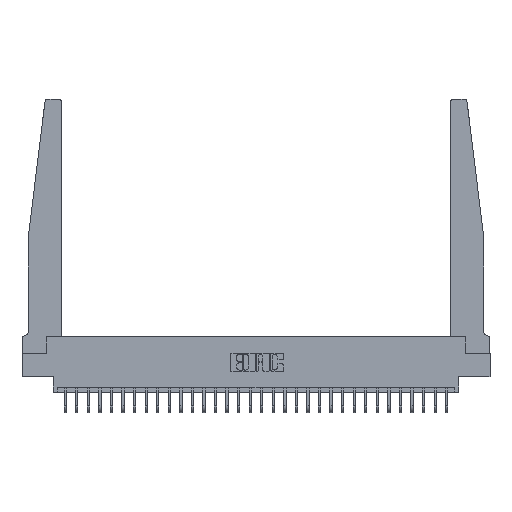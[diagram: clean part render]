
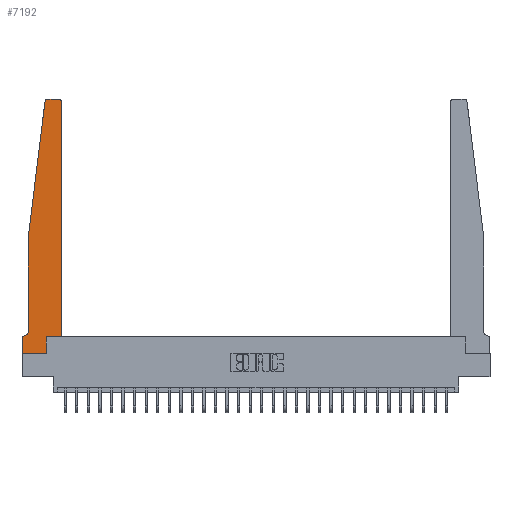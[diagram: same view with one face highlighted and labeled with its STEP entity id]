
A CAD part, top view. The second image highlights one B-rep face of the part: STEP entity #7192.
In plain terms, the highlighted planar face has unit normal (0, 0, 1).
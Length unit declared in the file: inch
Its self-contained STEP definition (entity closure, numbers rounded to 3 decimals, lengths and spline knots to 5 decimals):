
#477 = CARTESIAN_POINT ( 'NONE',  ( 0.425, 2.72, 0.37 ) ) ;
#1137 = CARTESIAN_POINT ( 'NONE',  ( 0.015, 0.2375, 0.37 ) ) ;
#1594 = VERTEX_POINT ( 'NONE', #477 ) ;
#1885 = CARTESIAN_POINT ( 'NONE',  ( 0., 0., 0.37 ) ) ;
#2144 = DIRECTION ( 'NONE',  ( 1., 0., 0. ) ) ;
#3073 = AXIS2_PLACEMENT_3D ( 'NONE', #11934, #12079, #19050 ) ;
#3601 = AXIS2_PLACEMENT_3D ( 'NONE', #6065, #6373, #27760 ) ;
#3822 = EDGE_CURVE ( 'NONE', #29778, #1594, #9329, .T. ) ;
#3919 = ORIENTED_EDGE ( 'NONE', *, *, #13113, .T. ) ;
#4171 = DIRECTION ( 'NONE',  ( -1., 0., 0. ) ) ;
#4250 = DIRECTION ( 'NONE',  ( 1., 0., 0. ) ) ;
#5122 = VERTEX_POINT ( 'NONE', #18334 ) ;
#5292 = DIRECTION ( 'NONE',  ( 0., -1., 0. ) ) ;
#5430 = DIRECTION ( 'NONE',  ( -1., 0., 0. ) ) ;
#5552 = CARTESIAN_POINT ( 'NONE',  ( 0.2605, 0.18, 0.37 ) ) ;
#5650 = ORIENTED_EDGE ( 'NONE', *, *, #11643, .T. ) ;
#5662 = VERTEX_POINT ( 'NONE', #12510 ) ;
#5674 = ORIENTED_EDGE ( 'NONE', *, *, #6452, .T. ) ;
#6065 = CARTESIAN_POINT ( 'NONE',  ( 0., 0.1875, 0.37 ) ) ;
#6373 = DIRECTION ( 'NONE',  ( 0., 0., 1. ) ) ;
#6452 = EDGE_CURVE ( 'NONE', #7779, #13140, #18598, .T. ) ;
#6862 = VECTOR ( 'NONE', #29755, 39.37008 ) ;
#7192 = ADVANCED_FACE ( 'NONE', ( #15463 ), #25291, .T. ) ;
#7197 = ORIENTED_EDGE ( 'NONE', *, *, #28856, .T. ) ;
#7530 = CARTESIAN_POINT ( 'NONE',  ( 0.015, 0.1875, 0.37 ) ) ;
#7582 = LINE ( 'NONE', #21440, #22960 ) ;
#7600 = EDGE_CURVE ( 'NONE', #5662, #25747, #27658, .T. ) ;
#7771 = LINE ( 'NONE', #12368, #23000 ) ;
#7779 = VERTEX_POINT ( 'NONE', #1885 ) ;
#7804 = ORIENTED_EDGE ( 'NONE', *, *, #14779, .T. ) ;
#7854 = ORIENTED_EDGE ( 'NONE', *, *, #20673, .T. ) ;
#8581 = VERTEX_POINT ( 'NONE', #29329 ) ;
#8921 = AXIS2_PLACEMENT_3D ( 'NONE', #9304, #21156, #4250 ) ;
#9181 = CARTESIAN_POINT ( 'NONE',  ( 0.425, 0.18, 0.37 ) ) ;
#9304 = CARTESIAN_POINT ( 'NONE',  ( 0.27653, 2.72, 0.37 ) ) ;
#9329 = LINE ( 'NONE', #9181, #12279 ) ;
#9482 = VECTOR ( 'NONE', #18603, 39.37008 ) ;
#10221 = DIRECTION ( 'NONE',  ( -0.122, -0.992, 0. ) ) ;
#11483 = DIRECTION ( 'NONE',  ( 0., 1., 0. ) ) ;
#11643 = EDGE_CURVE ( 'NONE', #14160, #29778, #25622, .T. ) ;
#11934 = CARTESIAN_POINT ( 'NONE',  ( 0.395, 2.72, 0.37 ) ) ;
#12009 = CARTESIAN_POINT ( 'NONE',  ( 0.27653, 2.75, 0.37 ) ) ;
#12079 = DIRECTION ( 'NONE',  ( 0., 0., 1. ) ) ;
#12270 = CARTESIAN_POINT ( 'NONE',  ( 0.425, 0.18, 0.37 ) ) ;
#12279 = VECTOR ( 'NONE', #11483, 39.37008 ) ;
#12280 = EDGE_CURVE ( 'NONE', #8581, #7779, #7582, .T. ) ;
#12368 = CARTESIAN_POINT ( 'NONE',  ( 0.065, 1.25, 0.37 ) ) ;
#12510 = CARTESIAN_POINT ( 'NONE',  ( 0.065, 0.2375, 0.37 ) ) ;
#13113 = EDGE_CURVE ( 'NONE', #5122, #15072, #7771, .T. ) ;
#13140 = VERTEX_POINT ( 'NONE', #21777 ) ;
#13266 = CARTESIAN_POINT ( 'NONE',  ( 0.065, 1.25, 0.37 ) ) ;
#13571 = LINE ( 'NONE', #13266, #6862 ) ;
#13627 = DIRECTION ( 'NONE',  ( 1., 0., 0. ) ) ;
#14160 = VERTEX_POINT ( 'NONE', #5552 ) ;
#14283 = ORIENTED_EDGE ( 'NONE', *, *, #19389, .T. ) ;
#14779 = EDGE_CURVE ( 'NONE', #15072, #5662, #13571, .T. ) ;
#15072 = VERTEX_POINT ( 'NONE', #29415 ) ;
#15253 = DIRECTION ( 'NONE',  ( -1., 0., 0. ) ) ;
#15385 = AXIS2_PLACEMENT_3D ( 'NONE', #1137, #21571, #5430 ) ;
#15463 = FACE_OUTER_BOUND ( 'NONE', #25776, .T. ) ;
#15940 = VECTOR ( 'NONE', #4171, 39.37008 ) ;
#17299 = ORIENTED_EDGE ( 'NONE', *, *, #3822, .T. ) ;
#18334 = CARTESIAN_POINT ( 'NONE',  ( 0.24675, 2.72367, 0.37 ) ) ;
#18484 = CARTESIAN_POINT ( 'NONE',  ( 0.25, 2.75, 0.37 ) ) ;
#18598 = LINE ( 'NONE', #23183, #21782 ) ;
#18603 = DIRECTION ( 'NONE',  ( 0., 1., 0. ) ) ;
#19050 = DIRECTION ( 'NONE',  ( 1., 0., 0. ) ) ;
#19389 = EDGE_CURVE ( 'NONE', #24106, #5122, #30079, .T. ) ;
#19422 = CARTESIAN_POINT ( 'NONE',  ( 0.065, 0.1875, 0.37 ) ) ;
#20254 = CIRCLE ( 'NONE', #3073, 0.03 ) ;
#20673 = EDGE_CURVE ( 'NONE', #13140, #14160, #29846, .T. ) ;
#21156 = DIRECTION ( 'NONE',  ( 0., 0., 1. ) ) ;
#21440 = CARTESIAN_POINT ( 'NONE',  ( 0., 0., 0.37 ) ) ;
#21571 = DIRECTION ( 'NONE',  ( 0., 0., -1. ) ) ;
#21777 = CARTESIAN_POINT ( 'NONE',  ( 0.2605, 0., 0.37 ) ) ;
#21782 = VECTOR ( 'NONE', #2144, 39.37008 ) ;
#21973 = ORIENTED_EDGE ( 'NONE', *, *, #12280, .T. ) ;
#22960 = VECTOR ( 'NONE', #5292, 39.37008 ) ;
#22986 = EDGE_CURVE ( 'NONE', #25747, #8581, #24163, .T. ) ;
#23000 = VECTOR ( 'NONE', #10221, 39.37008 ) ;
#23183 = CARTESIAN_POINT ( 'NONE',  ( 0., 0., 0.37 ) ) ;
#23496 = CARTESIAN_POINT ( 'NONE',  ( 0.395, 2.75, 0.37 ) ) ;
#24106 = VERTEX_POINT ( 'NONE', #12009 ) ;
#24163 = LINE ( 'NONE', #19422, #26702 ) ;
#24342 = EDGE_CURVE ( 'NONE', #26241, #24106, #25240, .T. ) ;
#24412 = VECTOR ( 'NONE', #13627, 39.37008 ) ;
#25209 = CARTESIAN_POINT ( 'NONE',  ( 0.2605, 0.18, 0.37 ) ) ;
#25240 = LINE ( 'NONE', #18484, #15940 ) ;
#25291 = PLANE ( 'NONE',  #3601 ) ;
#25622 = LINE ( 'NONE', #28098, #24412 ) ;
#25747 = VERTEX_POINT ( 'NONE', #7530 ) ;
#25776 = EDGE_LOOP ( 'NONE', ( #30084, #14283, #3919, #7804, #30237, #30287, #21973, #5674, #7854, #5650, #17299, #7197 ) ) ;
#26241 = VERTEX_POINT ( 'NONE', #23496 ) ;
#26702 = VECTOR ( 'NONE', #15253, 39.37008 ) ;
#27658 = CIRCLE ( 'NONE', #15385, 0.05 ) ;
#27760 = DIRECTION ( 'NONE',  ( 1., 0., 0. ) ) ;
#28098 = CARTESIAN_POINT ( 'NONE',  ( 0.425, 0.18, 0.37 ) ) ;
#28856 = EDGE_CURVE ( 'NONE', #1594, #26241, #20254, .T. ) ;
#29329 = CARTESIAN_POINT ( 'NONE',  ( 0., 0.1875, 0.37 ) ) ;
#29415 = CARTESIAN_POINT ( 'NONE',  ( 0.065, 1.25, 0.37 ) ) ;
#29755 = DIRECTION ( 'NONE',  ( 0., -1., 0. ) ) ;
#29778 = VERTEX_POINT ( 'NONE', #12270 ) ;
#29846 = LINE ( 'NONE', #25209, #9482 ) ;
#30079 = CIRCLE ( 'NONE', #8921, 0.03 ) ;
#30084 = ORIENTED_EDGE ( 'NONE', *, *, #24342, .T. ) ;
#30237 = ORIENTED_EDGE ( 'NONE', *, *, #7600, .T. ) ;
#30287 = ORIENTED_EDGE ( 'NONE', *, *, #22986, .T. ) ;
